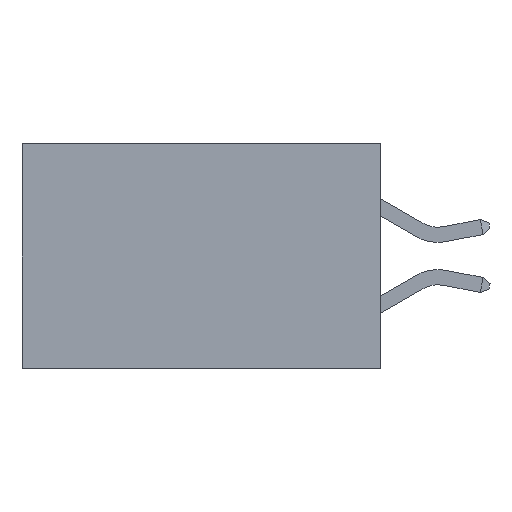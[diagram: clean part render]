
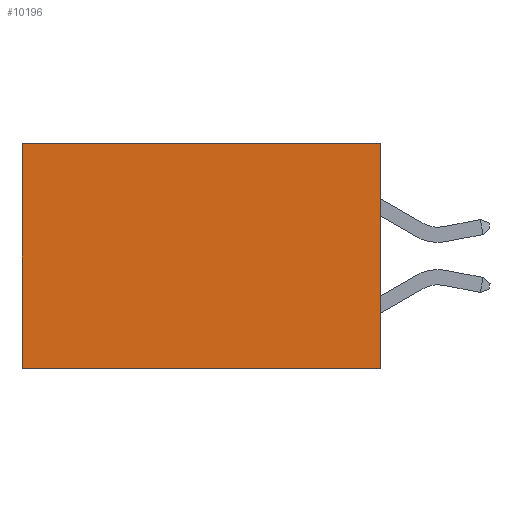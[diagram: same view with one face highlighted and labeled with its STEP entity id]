
A CAD part, left-side view. The second image highlights one B-rep face of the part: STEP entity #10196.
In plain terms, the highlighted planar face has unit normal (-1, 0, 0).
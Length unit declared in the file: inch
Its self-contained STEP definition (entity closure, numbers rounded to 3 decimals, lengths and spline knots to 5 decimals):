
#4 = DIRECTION ( 'NONE',  ( 0., 1., 0. ) ) ;
#105 = ORIENTED_EDGE ( 'NONE', *, *, #8014, .F. ) ;
#613 = CARTESIAN_POINT ( 'NONE',  ( 0.277, 0., -0.37 ) ) ;
#1542 = ORIENTED_EDGE ( 'NONE', *, *, #8466, .F. ) ;
#1735 = CARTESIAN_POINT ( 'NONE',  ( 0.277, 0., -0.37 ) ) ;
#1750 = VECTOR ( 'NONE', #13170, 39.37008 ) ;
#2104 = VECTOR ( 'NONE', #19852, 39.37008 ) ;
#5002 = DIRECTION ( 'NONE',  ( 0., 0., -1. ) ) ;
#5130 = DIRECTION ( 'NONE',  ( 1., 0., 0. ) ) ;
#5215 = CARTESIAN_POINT ( 'NONE',  ( 0.277, 0., -0.37 ) ) ;
#5245 = PLANE ( 'NONE',  #16199 ) ;
#6032 = LINE ( 'NONE', #8279, #11588 ) ;
#8014 = EDGE_CURVE ( 'NONE', #10471, #20406, #11614, .T. ) ;
#8279 = CARTESIAN_POINT ( 'NONE',  ( 0.277, 0., -0.37 ) ) ;
#8370 = LINE ( 'NONE', #25873, #2104 ) ;
#8466 = EDGE_CURVE ( 'NONE', #21100, #10471, #6032, .T. ) ;
#9813 = DIRECTION ( 'NONE',  ( 0., 0., -1. ) ) ;
#10196 = ADVANCED_FACE ( 'NONE', ( #25264 ), #5245, .F. ) ;
#10471 = VERTEX_POINT ( 'NONE', #1735 ) ;
#10841 = ORIENTED_EDGE ( 'NONE', *, *, #18884, .T. ) ;
#11588 = VECTOR ( 'NONE', #9813, 39.37008 ) ;
#11614 = LINE ( 'NONE', #613, #15719 ) ;
#11990 = CARTESIAN_POINT ( 'NONE',  ( 0.277, 0., 0. ) ) ;
#13170 = DIRECTION ( 'NONE',  ( 0., 1., 0. ) ) ;
#15184 = CARTESIAN_POINT ( 'NONE',  ( 0.277, 0., 0. ) ) ;
#15719 = VECTOR ( 'NONE', #4, 39.37008 ) ;
#16199 = AXIS2_PLACEMENT_3D ( 'NONE', #5215, #5130, #5002 ) ;
#18512 = ORIENTED_EDGE ( 'NONE', *, *, #24705, .T. ) ;
#18884 = EDGE_CURVE ( 'NONE', #24403, #20406, #8370, .T. ) ;
#19852 = DIRECTION ( 'NONE',  ( 0., 0., -1. ) ) ;
#20339 = CARTESIAN_POINT ( 'NONE',  ( 0.277, 0.59, 0. ) ) ;
#20406 = VERTEX_POINT ( 'NONE', #23951 ) ;
#21100 = VERTEX_POINT ( 'NONE', #11990 ) ;
#22180 = EDGE_LOOP ( 'NONE', ( #10841, #105, #1542, #18512 ) ) ;
#23503 = LINE ( 'NONE', #15184, #1750 ) ;
#23951 = CARTESIAN_POINT ( 'NONE',  ( 0.277, 0.59, -0.37 ) ) ;
#24403 = VERTEX_POINT ( 'NONE', #20339 ) ;
#24705 = EDGE_CURVE ( 'NONE', #21100, #24403, #23503, .T. ) ;
#25264 = FACE_OUTER_BOUND ( 'NONE', #22180, .T. ) ;
#25873 = CARTESIAN_POINT ( 'NONE',  ( 0.277, 0.59, -0.37 ) ) ;
